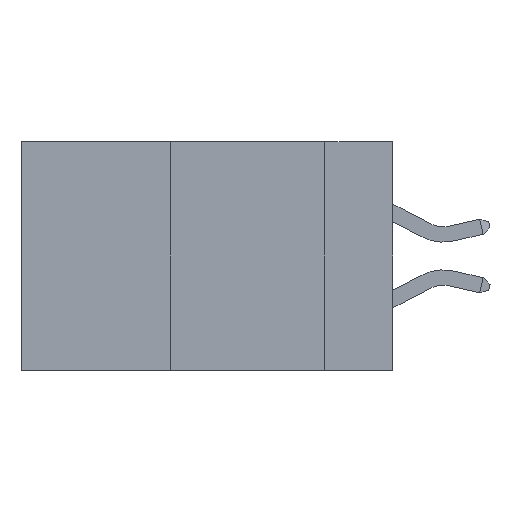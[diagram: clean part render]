
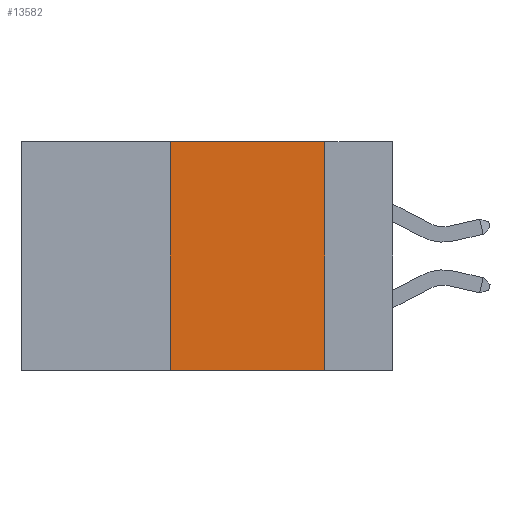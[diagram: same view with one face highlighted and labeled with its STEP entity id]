
A CAD part, left-side view. The second image highlights one B-rep face of the part: STEP entity #13582.
In plain terms, the highlighted planar face has unit normal (-1, 0, 0).
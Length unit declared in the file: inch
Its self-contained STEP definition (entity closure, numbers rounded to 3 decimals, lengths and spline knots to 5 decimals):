
#780 = CARTESIAN_POINT ( 'NONE',  ( 0., 0.6, 0. ) ) ;
#1187 = ORIENTED_EDGE ( 'NONE', *, *, #15839, .F. ) ;
#1271 = DIRECTION ( 'NONE',  ( 0., 0., -1. ) ) ;
#1274 = LINE ( 'NONE', #10394, #14049 ) ;
#1590 = VERTEX_POINT ( 'NONE', #8160 ) ;
#2165 = AXIS2_PLACEMENT_3D ( 'NONE', #22005, #20313, #9703 ) ;
#3753 = LINE ( 'NONE', #780, #22194 ) ;
#4229 = PLANE ( 'NONE',  #2165 ) ;
#4865 = LINE ( 'NONE', #10324, #9701 ) ;
#5262 = VECTOR ( 'NONE', #9799, 39.37008 ) ;
#5411 = EDGE_CURVE ( 'NONE', #10060, #6608, #15399, .T. ) ;
#6247 = CARTESIAN_POINT ( 'NONE',  ( 0., 0.36, 0. ) ) ;
#6608 = VERTEX_POINT ( 'NONE', #22449 ) ;
#8160 = CARTESIAN_POINT ( 'NONE',  ( 0., 0.11, -0.37 ) ) ;
#8421 = FACE_OUTER_BOUND ( 'NONE', #20749, .T. ) ;
#9701 = VECTOR ( 'NONE', #12108, 39.37008 ) ;
#9703 = DIRECTION ( 'NONE',  ( 0., 0., -1. ) ) ;
#9799 = DIRECTION ( 'NONE',  ( 0., 0., 1. ) ) ;
#10060 = VERTEX_POINT ( 'NONE', #22294 ) ;
#10324 = CARTESIAN_POINT ( 'NONE',  ( 0., 0.6, -0.37 ) ) ;
#10394 = CARTESIAN_POINT ( 'NONE',  ( 0., 0.11, 0. ) ) ;
#12108 = DIRECTION ( 'NONE',  ( 0., -1., 0. ) ) ;
#12570 = ORIENTED_EDGE ( 'NONE', *, *, #22592, .T. ) ;
#13548 = VERTEX_POINT ( 'NONE', #18467 ) ;
#13582 = ADVANCED_FACE ( 'NONE', ( #8421 ), #4229, .F. ) ;
#14049 = VECTOR ( 'NONE', #1271, 39.37008 ) ;
#15399 = LINE ( 'NONE', #6247, #5262 ) ;
#15839 = EDGE_CURVE ( 'NONE', #6608, #13548, #3753, .T. ) ;
#17088 = DIRECTION ( 'NONE',  ( 0., -1., 0. ) ) ;
#18467 = CARTESIAN_POINT ( 'NONE',  ( 0., 0.11, 0. ) ) ;
#18606 = EDGE_CURVE ( 'NONE', #13548, #1590, #1274, .T. ) ;
#18666 = ORIENTED_EDGE ( 'NONE', *, *, #18606, .F. ) ;
#20313 = DIRECTION ( 'NONE',  ( 1., 0., 0. ) ) ;
#20318 = ORIENTED_EDGE ( 'NONE', *, *, #5411, .F. ) ;
#20749 = EDGE_LOOP ( 'NONE', ( #18666, #1187, #20318, #12570 ) ) ;
#22005 = CARTESIAN_POINT ( 'NONE',  ( 0., 0.6, 0. ) ) ;
#22194 = VECTOR ( 'NONE', #17088, 39.37008 ) ;
#22294 = CARTESIAN_POINT ( 'NONE',  ( 0., 0.36, -0.37 ) ) ;
#22449 = CARTESIAN_POINT ( 'NONE',  ( 0., 0.36, 0. ) ) ;
#22592 = EDGE_CURVE ( 'NONE', #10060, #1590, #4865, .T. ) ;
